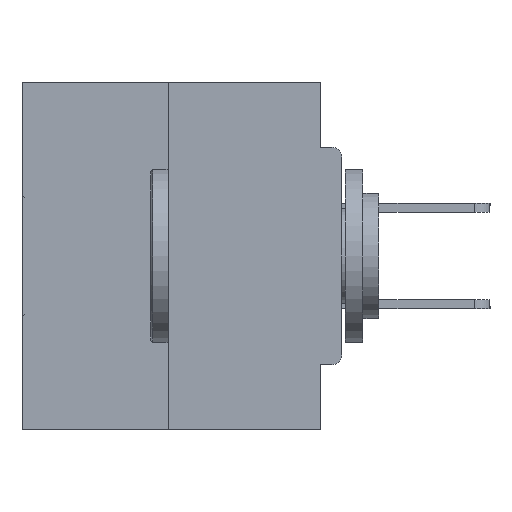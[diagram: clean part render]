
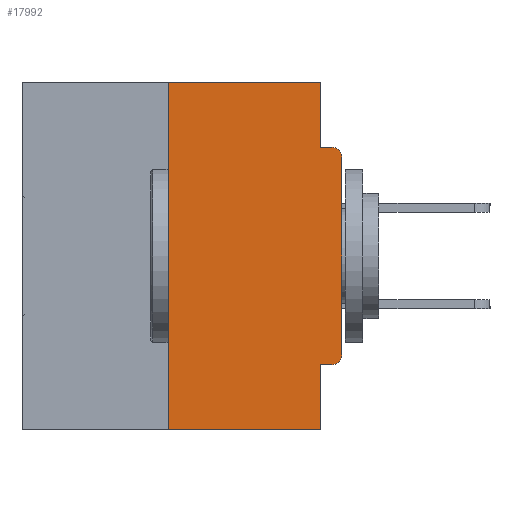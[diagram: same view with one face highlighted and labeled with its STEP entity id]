
A CAD part, left-side view. The second image highlights one B-rep face of the part: STEP entity #17992.
In plain terms, the highlighted planar face has unit normal (-1, 0, 0).
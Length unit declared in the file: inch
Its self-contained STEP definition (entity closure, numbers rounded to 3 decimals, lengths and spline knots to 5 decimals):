
#704 = LINE ( 'NONE', #1193, #40383 ) ;
#758 = CARTESIAN_POINT ( 'NONE',  ( 0., 0.25, -0.5 ) ) ;
#1122 = VERTEX_POINT ( 'NONE', #22846 ) ;
#1193 = CARTESIAN_POINT ( 'NONE',  ( 0., 0.031, 0. ) ) ;
#1762 = FACE_OUTER_BOUND ( 'NONE', #15714, .T. ) ;
#2734 = VERTEX_POINT ( 'NONE', #758 ) ;
#3112 = VECTOR ( 'NONE', #10787, 39.37008 ) ;
#3180 = LINE ( 'NONE', #8338, #40373 ) ;
#4258 = VECTOR ( 'NONE', #5245, 39.37008 ) ;
#5085 = DIRECTION ( 'NONE',  ( 0., 0., -1. ) ) ;
#5245 = DIRECTION ( 'NONE',  ( 0., -1., 0. ) ) ;
#5373 = LINE ( 'NONE', #27888, #18420 ) ;
#6123 = CARTESIAN_POINT ( 'NONE',  ( 0., 0.015, -0.3915 ) ) ;
#6150 = CARTESIAN_POINT ( 'NONE',  ( 0., 0.46, 0. ) ) ;
#6326 = CARTESIAN_POINT ( 'NONE',  ( 0., 0., -0.3915 ) ) ;
#7052 = ORIENTED_EDGE ( 'NONE', *, *, #28080, .F. ) ;
#7801 = ORIENTED_EDGE ( 'NONE', *, *, #34074, .T. ) ;
#7999 = ORIENTED_EDGE ( 'NONE', *, *, #9682, .T. ) ;
#8338 = CARTESIAN_POINT ( 'NONE',  ( 0., 0., 0. ) ) ;
#8450 = ORIENTED_EDGE ( 'NONE', *, *, #19042, .T. ) ;
#8475 = CARTESIAN_POINT ( 'NONE',  ( 0., 0., -0.4065 ) ) ;
#8486 = VERTEX_POINT ( 'NONE', #28912 ) ;
#9408 = DIRECTION ( 'NONE',  ( 1., 0., 0. ) ) ;
#9682 = EDGE_CURVE ( 'NONE', #11683, #36254, #33784, .T. ) ;
#9683 = DIRECTION ( 'NONE',  ( 0., 0., -1. ) ) ;
#10730 = VERTEX_POINT ( 'NONE', #11980 ) ;
#10787 = DIRECTION ( 'NONE',  ( 0., 1., 0. ) ) ;
#10900 = CARTESIAN_POINT ( 'NONE',  ( 0., 0.031, -0.5 ) ) ;
#11048 = LINE ( 'NONE', #10900, #17497 ) ;
#11683 = VERTEX_POINT ( 'NONE', #12780 ) ;
#11980 = CARTESIAN_POINT ( 'NONE',  ( 0., 0.031, -0.5 ) ) ;
#12780 = CARTESIAN_POINT ( 'NONE',  ( 0., 0., -0.1085 ) ) ;
#13183 = AXIS2_PLACEMENT_3D ( 'NONE', #6123, #15761, #22263 ) ;
#14756 = CARTESIAN_POINT ( 'NONE',  ( 0., 0.46, -0.5 ) ) ;
#15635 = CARTESIAN_POINT ( 'NONE',  ( 0., 0., -0.0935 ) ) ;
#15714 = EDGE_LOOP ( 'NONE', ( #19741, #31644, #20006, #29313, #32283, #7801, #8450, #7999, #7052, #25338 ) ) ;
#15761 = DIRECTION ( 'NONE',  ( -1., 0., 0. ) ) ;
#16150 = LINE ( 'NONE', #8475, #3112 ) ;
#16196 = LINE ( 'NONE', #15635, #25236 ) ;
#16269 = EDGE_CURVE ( 'NONE', #27448, #23818, #16150, .T. ) ;
#16561 = CARTESIAN_POINT ( 'NONE',  ( 0., 0.015, -0.4065 ) ) ;
#16615 = CARTESIAN_POINT ( 'NONE',  ( 0., 0.031, -0.4065 ) ) ;
#16723 = EDGE_CURVE ( 'NONE', #23818, #10730, #11048, .T. ) ;
#17339 = EDGE_CURVE ( 'NONE', #8486, #39580, #5373, .T. ) ;
#17497 = VECTOR ( 'NONE', #23622, 39.37008 ) ;
#17992 = ADVANCED_FACE ( 'NONE', ( #1762 ), #22008, .F. ) ;
#18221 = CARTESIAN_POINT ( 'NONE',  ( 0., 0.031, 0. ) ) ;
#18223 = CARTESIAN_POINT ( 'NONE',  ( 0., 0.25, 0. ) ) ;
#18420 = VECTOR ( 'NONE', #34090, 39.37008 ) ;
#18693 = EDGE_CURVE ( 'NONE', #2734, #10730, #29879, .T. ) ;
#19042 = EDGE_CURVE ( 'NONE', #41482, #11683, #3180, .T. ) ;
#19741 = ORIENTED_EDGE ( 'NONE', *, *, #17339, .F. ) ;
#20006 = ORIENTED_EDGE ( 'NONE', *, *, #18693, .T. ) ;
#21636 = AXIS2_PLACEMENT_3D ( 'NONE', #6150, #9408, #9683 ) ;
#22008 = PLANE ( 'NONE',  #21636 ) ;
#22263 = DIRECTION ( 'NONE',  ( 0., 0., -1. ) ) ;
#22846 = CARTESIAN_POINT ( 'NONE',  ( 0., 0.031, -0.0935 ) ) ;
#23622 = DIRECTION ( 'NONE',  ( 0., 0., -1. ) ) ;
#23818 = VERTEX_POINT ( 'NONE', #16615 ) ;
#24000 = CIRCLE ( 'NONE', #13183, 0.015 ) ;
#24818 = DIRECTION ( 'NONE',  ( 0., 0., 1. ) ) ;
#25236 = VECTOR ( 'NONE', #41338, 39.37008 ) ;
#25338 = ORIENTED_EDGE ( 'NONE', *, *, #26944, .F. ) ;
#26923 = LINE ( 'NONE', #18223, #38961 ) ;
#26944 = EDGE_CURVE ( 'NONE', #39580, #1122, #704, .T. ) ;
#27024 = DIRECTION ( 'NONE',  ( 0., 0., 1. ) ) ;
#27448 = VERTEX_POINT ( 'NONE', #16561 ) ;
#27888 = CARTESIAN_POINT ( 'NONE',  ( 0., 0.46, 0. ) ) ;
#28080 = EDGE_CURVE ( 'NONE', #1122, #36254, #16196, .T. ) ;
#28912 = CARTESIAN_POINT ( 'NONE',  ( 0., 0.25, 0. ) ) ;
#29313 = ORIENTED_EDGE ( 'NONE', *, *, #16723, .F. ) ;
#29879 = LINE ( 'NONE', #14756, #4258 ) ;
#31644 = ORIENTED_EDGE ( 'NONE', *, *, #37781, .F. ) ;
#32283 = ORIENTED_EDGE ( 'NONE', *, *, #16269, .F. ) ;
#33654 = DIRECTION ( 'NONE',  ( 0., 0., -1. ) ) ;
#33784 = CIRCLE ( 'NONE', #36496, 0.015 ) ;
#34074 = EDGE_CURVE ( 'NONE', #27448, #41482, #24000, .T. ) ;
#34090 = DIRECTION ( 'NONE',  ( 0., -1., 0. ) ) ;
#34176 = CARTESIAN_POINT ( 'NONE',  ( 0., 0.015, -0.0935 ) ) ;
#36254 = VERTEX_POINT ( 'NONE', #34176 ) ;
#36496 = AXIS2_PLACEMENT_3D ( 'NONE', #40716, #40455, #5085 ) ;
#37781 = EDGE_CURVE ( 'NONE', #2734, #8486, #26923, .T. ) ;
#38961 = VECTOR ( 'NONE', #24818, 39.37008 ) ;
#39580 = VERTEX_POINT ( 'NONE', #18221 ) ;
#40373 = VECTOR ( 'NONE', #27024, 39.37008 ) ;
#40383 = VECTOR ( 'NONE', #33654, 39.37008 ) ;
#40455 = DIRECTION ( 'NONE',  ( -1., 0., 0. ) ) ;
#40716 = CARTESIAN_POINT ( 'NONE',  ( 0., 0.015, -0.1085 ) ) ;
#41338 = DIRECTION ( 'NONE',  ( 0., -1., 0. ) ) ;
#41482 = VERTEX_POINT ( 'NONE', #6326 ) ;
